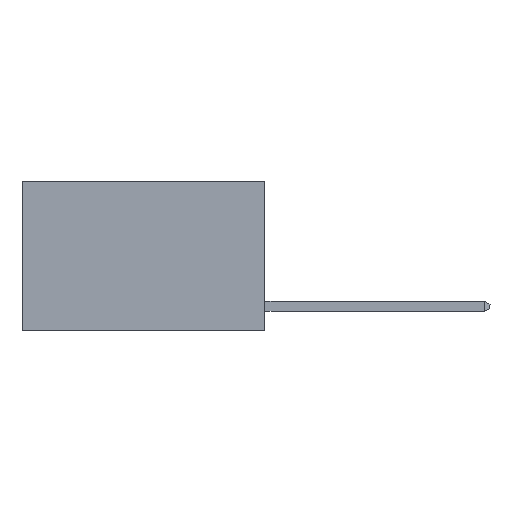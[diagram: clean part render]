
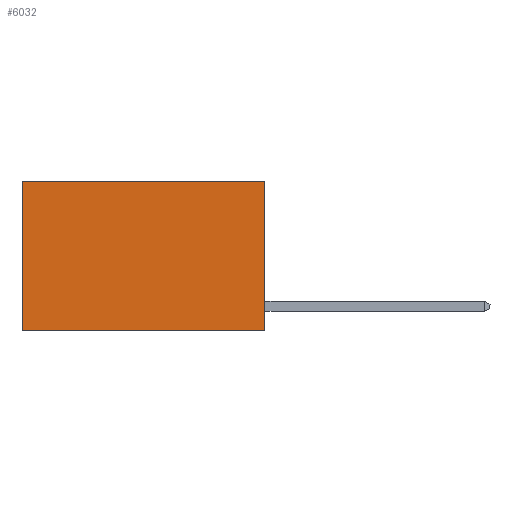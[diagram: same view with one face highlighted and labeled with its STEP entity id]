
A CAD part, left-side view. The second image highlights one B-rep face of the part: STEP entity #6032.
In plain terms, the highlighted planar face has unit normal (-1, 0, 0).
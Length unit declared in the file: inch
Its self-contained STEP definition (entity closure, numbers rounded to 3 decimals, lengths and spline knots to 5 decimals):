
#25 = EDGE_CURVE ( 'NONE', #1433, #2432, #11368, .T. ) ;
#60 = DIRECTION ( 'NONE',  ( 0., 0., -1. ) ) ;
#240 = CARTESIAN_POINT ( 'NONE',  ( 0.2625, 0., 0. ) ) ;
#364 = ORIENTED_EDGE ( 'NONE', *, *, #25, .F. ) ;
#507 = DIRECTION ( 'NONE',  ( 1., 0., 0. ) ) ;
#915 = ORIENTED_EDGE ( 'NONE', *, *, #11594, .F. ) ;
#1433 = VERTEX_POINT ( 'NONE', #2718 ) ;
#1488 = ORIENTED_EDGE ( 'NONE', *, *, #6272, .T. ) ;
#2432 = VERTEX_POINT ( 'NONE', #10292 ) ;
#2718 = CARTESIAN_POINT ( 'NONE',  ( 0.2625, 0., -0.37 ) ) ;
#3567 = VECTOR ( 'NONE', #9674, 39.37008 ) ;
#3741 = VECTOR ( 'NONE', #60, 39.37008 ) ;
#4010 = LINE ( 'NONE', #10934, #3741 ) ;
#4292 = CARTESIAN_POINT ( 'NONE',  ( 0.2625, 0.6, 0. ) ) ;
#5824 = PLANE ( 'NONE',  #11395 ) ;
#6032 = ADVANCED_FACE ( 'NONE', ( #9107 ), #5824, .F. ) ;
#6272 = EDGE_CURVE ( 'NONE', #9424, #9732, #6396, .T. ) ;
#6396 = LINE ( 'NONE', #240, #11301 ) ;
#6508 = DIRECTION ( 'NONE',  ( 0., 1., 0. ) ) ;
#6780 = CARTESIAN_POINT ( 'NONE',  ( 0.2625, 0., 0. ) ) ;
#6828 = DIRECTION ( 'NONE',  ( 0., 0., -1. ) ) ;
#7062 = CARTESIAN_POINT ( 'NONE',  ( 0.2625, 0., -0.37 ) ) ;
#8766 = CARTESIAN_POINT ( 'NONE',  ( 0.2625, 0.6, 0. ) ) ;
#9046 = VECTOR ( 'NONE', #9828, 39.37008 ) ;
#9107 = FACE_OUTER_BOUND ( 'NONE', #10189, .T. ) ;
#9137 = LINE ( 'NONE', #8766, #3567 ) ;
#9227 = ORIENTED_EDGE ( 'NONE', *, *, #10359, .T. ) ;
#9424 = VERTEX_POINT ( 'NONE', #10487 ) ;
#9674 = DIRECTION ( 'NONE',  ( 0., 0., -1. ) ) ;
#9732 = VERTEX_POINT ( 'NONE', #4292 ) ;
#9828 = DIRECTION ( 'NONE',  ( 0., 1., 0. ) ) ;
#10189 = EDGE_LOOP ( 'NONE', ( #9227, #364, #915, #1488 ) ) ;
#10292 = CARTESIAN_POINT ( 'NONE',  ( 0.2625, 0.6, -0.37 ) ) ;
#10359 = EDGE_CURVE ( 'NONE', #9732, #2432, #9137, .T. ) ;
#10487 = CARTESIAN_POINT ( 'NONE',  ( 0.2625, 0., 0. ) ) ;
#10934 = CARTESIAN_POINT ( 'NONE',  ( 0.2625, 0., 0. ) ) ;
#11301 = VECTOR ( 'NONE', #6508, 39.37008 ) ;
#11368 = LINE ( 'NONE', #7062, #9046 ) ;
#11395 = AXIS2_PLACEMENT_3D ( 'NONE', #6780, #507, #6828 ) ;
#11594 = EDGE_CURVE ( 'NONE', #9424, #1433, #4010, .T. ) ;
